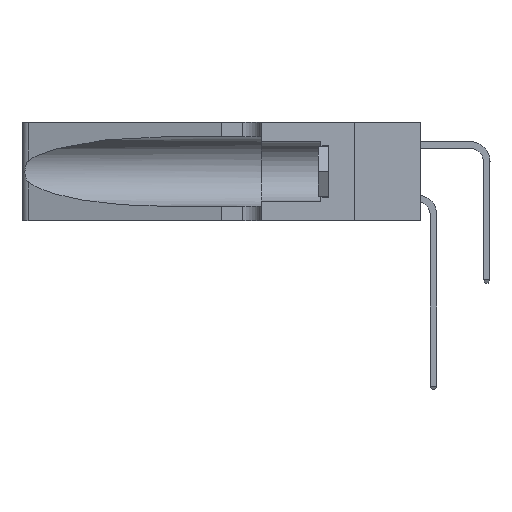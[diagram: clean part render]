
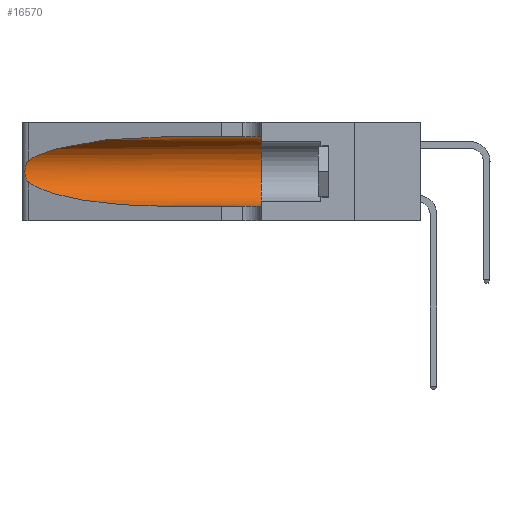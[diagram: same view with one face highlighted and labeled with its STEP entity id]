
A CAD part, left-side view. The second image highlights one B-rep face of the part: STEP entity #16570.
In plain terms, the highlighted cylindrical face has radius 3.308 mm (diameter 6.617 mm), a partial arc.
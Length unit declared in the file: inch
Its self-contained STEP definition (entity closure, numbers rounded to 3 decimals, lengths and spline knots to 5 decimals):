
#1436 = ORIENTED_EDGE ( 'NONE', *, *, #21552, .T. ) ;
#1501 = CARTESIAN_POINT ( 'NONE',  ( 0.25487, 1.22718, 0.22369 ) ) ;
#1570 =( BOUNDED_CURVE ( )  B_SPLINE_CURVE ( 3, ( #4227, #21531, #13026, #2574 ),
 .UNSPECIFIED., .F., .F. ) 
 B_SPLINE_CURVE_WITH_KNOTS ( ( 4, 4 ),
 ( 3.44316, 4.71239 ),
 .UNSPECIFIED. ) 
 CURVE ( )  GEOMETRIC_REPRESENTATION_ITEM ( )  RATIONAL_B_SPLINE_CURVE ( ( 1., 0.87, 0.87, 1. ) ) 
 REPRESENTATION_ITEM ( '' )  );
#1657 = EDGE_LOOP ( 'NONE', ( #4964, #18811, #1436, #10760, #7194, #20933 ) ) ;
#1922 = VERTEX_POINT ( 'NONE', #19142 ) ;
#2153 = B_SPLINE_CURVE_WITH_KNOTS ( 'NONE', 3,
 ( #11526, #20063, #13266, #2813, #15000, #4529, #16719, #6313, #18419, #8083, #20131, #9830, #21834, #11602 ),
 .UNSPECIFIED., .F., .F.,
 ( 4, 2, 2, 2, 2, 2, 4 ),
 ( 0., 0.00027, 0.00053, 0.00107, 0.0016, 0.00187, 0.00214 ),
 .UNSPECIFIED. ) ;
#2574 = CARTESIAN_POINT ( 'NONE',  ( 0.1305, 0.72297, 0.05475 ) ) ;
#2813 = CARTESIAN_POINT ( 'NONE',  ( 0.25787, 1.23484, 0.2124 ) ) ;
#2868 =( BOUNDED_CURVE ( )  B_SPLINE_CURVE ( 3, ( #11996, #22220, #3116, #1501 ),
 .UNSPECIFIED., .F., .F. ) 
 B_SPLINE_CURVE_WITH_KNOTS ( ( 4, 4 ),
 ( 1.5708, 2.84003 ),
 .UNSPECIFIED. ) 
 CURVE ( )  GEOMETRIC_REPRESENTATION_ITEM ( )  RATIONAL_B_SPLINE_CURVE ( ( 1., 0.87, 0.87, 1. ) ) 
 REPRESENTATION_ITEM ( '' )  );
#3116 = CARTESIAN_POINT ( 'NONE',  ( 0.2373, 1.15595, 0.28018 ) ) ;
#3789 = CARTESIAN_POINT ( 'NONE',  ( 0.1305, 1.61858, 0.31525 ) ) ;
#3945 = CARTESIAN_POINT ( 'NONE',  ( 0.1305, 0.72297, 0.31525 ) ) ;
#4130 = LINE ( 'NONE', #3789, #17983 ) ;
#4227 = CARTESIAN_POINT ( 'NONE',  ( 0.25487, 1.22718, 0.14631 ) ) ;
#4529 = CARTESIAN_POINT ( 'NONE',  ( 0.26018, 1.23835, 0.19895 ) ) ;
#4754 = VERTEX_POINT ( 'NONE', #18690 ) ;
#4964 = ORIENTED_EDGE ( 'NONE', *, *, #14720, .T. ) ;
#5572 = CARTESIAN_POINT ( 'NONE',  ( 0.1305, 1.61858, 0.05475 ) ) ;
#6313 = CARTESIAN_POINT ( 'NONE',  ( 0.26075, 1.23896, 0.178 ) ) ;
#6423 = CYLINDRICAL_SURFACE ( 'NONE', #17506, 0.13025 ) ;
#6565 = CIRCLE ( 'NONE', #19514, 0.13025 ) ;
#7194 = ORIENTED_EDGE ( 'NONE', *, *, #18527, .F. ) ;
#7219 = CARTESIAN_POINT ( 'NONE',  ( 0.1305, 0.35, 0.185 ) ) ;
#7849 = CARTESIAN_POINT ( 'NONE',  ( 0.25487, 1.22718, 0.22369 ) ) ;
#8083 = CARTESIAN_POINT ( 'NONE',  ( 0.25856, 1.23593, 0.16098 ) ) ;
#8979 = DIRECTION ( 'NONE',  ( 0., 0., 1. ) ) ;
#8990 = VERTEX_POINT ( 'NONE', #17898 ) ;
#9830 = CARTESIAN_POINT ( 'NONE',  ( 0.25639, 1.23186, 0.15144 ) ) ;
#10760 = ORIENTED_EDGE ( 'NONE', *, *, #13637, .T. ) ;
#11526 = CARTESIAN_POINT ( 'NONE',  ( 0.25487, 1.22718, 0.22369 ) ) ;
#11602 = CARTESIAN_POINT ( 'NONE',  ( 0.25487, 1.22718, 0.14631 ) ) ;
#11852 = DIRECTION ( 'NONE',  ( 0., -1., 0. ) ) ;
#11996 = CARTESIAN_POINT ( 'NONE',  ( 0.1305, 0.72297, 0.31525 ) ) ;
#12498 = EDGE_CURVE ( 'NONE', #20761, #1922, #4130, .T. ) ;
#13003 = CARTESIAN_POINT ( 'NONE',  ( 0.25487, 1.22718, 0.14631 ) ) ;
#13026 = CARTESIAN_POINT ( 'NONE',  ( 0.18966, 0.96281, 0.05475 ) ) ;
#13266 = CARTESIAN_POINT ( 'NONE',  ( 0.25639, 1.23184, 0.21858 ) ) ;
#13637 = EDGE_CURVE ( 'NONE', #4754, #8990, #16062, .T. ) ;
#14484 = DIRECTION ( 'NONE',  ( 0., -1., 0. ) ) ;
#14720 = EDGE_CURVE ( 'NONE', #20761, #16936, #2868, .T. ) ;
#15000 = CARTESIAN_POINT ( 'NONE',  ( 0.25854, 1.2359, 0.20912 ) ) ;
#15700 = VERTEX_POINT ( 'NONE', #13003 ) ;
#16062 = LINE ( 'NONE', #5572, #20589 ) ;
#16570 = ADVANCED_FACE ( 'NONE', ( #20196 ), #6423, .F. ) ;
#16719 = CARTESIAN_POINT ( 'NONE',  ( 0.26075, 1.23896, 0.19203 ) ) ;
#16936 = VERTEX_POINT ( 'NONE', #7849 ) ;
#17506 = AXIS2_PLACEMENT_3D ( 'NONE', #22068, #11852, #18583 ) ;
#17898 = CARTESIAN_POINT ( 'NONE',  ( 0.1305, 0.35, 0.05475 ) ) ;
#17983 = VECTOR ( 'NONE', #14484, 39.37008 ) ;
#18228 = EDGE_CURVE ( 'NONE', #16936, #15700, #2153, .T. ) ;
#18419 = CARTESIAN_POINT ( 'NONE',  ( 0.26017, 1.23833, 0.17102 ) ) ;
#18527 = EDGE_CURVE ( 'NONE', #1922, #8990, #6565, .T. ) ;
#18583 = DIRECTION ( 'NONE',  ( 0., 0., -1. ) ) ;
#18690 = CARTESIAN_POINT ( 'NONE',  ( 0.1305, 0.72297, 0.05475 ) ) ;
#18811 = ORIENTED_EDGE ( 'NONE', *, *, #18228, .T. ) ;
#19142 = CARTESIAN_POINT ( 'NONE',  ( 0.1305, 0.35, 0.31525 ) ) ;
#19282 = DIRECTION ( 'NONE',  ( 0., 1., 0. ) ) ;
#19514 = AXIS2_PLACEMENT_3D ( 'NONE', #7219, #19282, #8979 ) ;
#20063 = CARTESIAN_POINT ( 'NONE',  ( 0.25555, 1.22994, 0.2215 ) ) ;
#20131 = CARTESIAN_POINT ( 'NONE',  ( 0.25789, 1.23486, 0.15765 ) ) ;
#20196 = FACE_OUTER_BOUND ( 'NONE', #1657, .T. ) ;
#20589 = VECTOR ( 'NONE', #21134, 39.37008 ) ;
#20761 = VERTEX_POINT ( 'NONE', #3945 ) ;
#20933 = ORIENTED_EDGE ( 'NONE', *, *, #12498, .F. ) ;
#21134 = DIRECTION ( 'NONE',  ( 0., -1., 0. ) ) ;
#21531 = CARTESIAN_POINT ( 'NONE',  ( 0.2373, 1.15595, 0.08982 ) ) ;
#21552 = EDGE_CURVE ( 'NONE', #15700, #4754, #1570, .T. ) ;
#21834 = CARTESIAN_POINT ( 'NONE',  ( 0.25555, 1.22993, 0.14849 ) ) ;
#22068 = CARTESIAN_POINT ( 'NONE',  ( 0.1305, 1.61858, 0.185 ) ) ;
#22220 = CARTESIAN_POINT ( 'NONE',  ( 0.18966, 0.96281, 0.31525 ) ) ;
